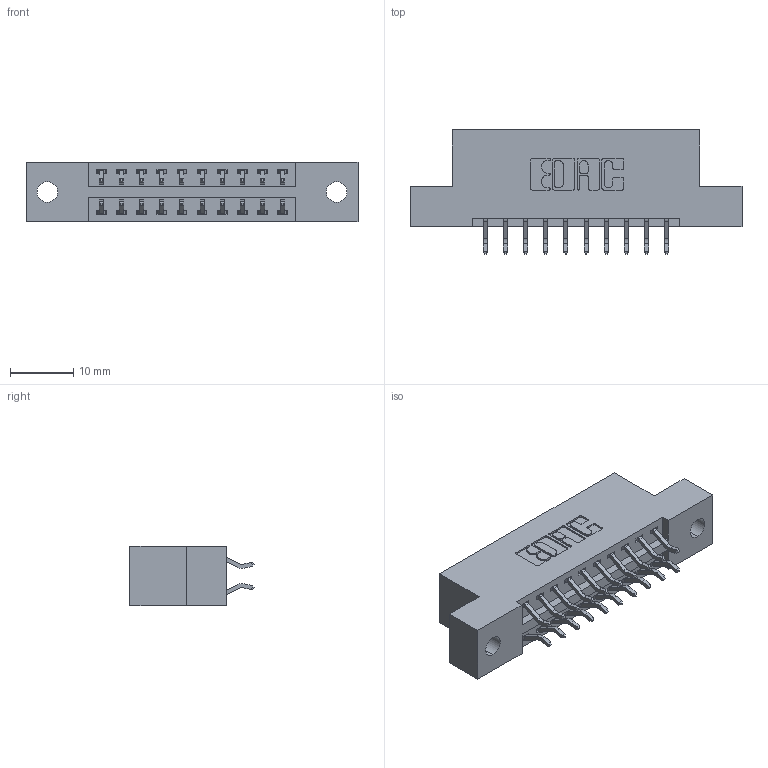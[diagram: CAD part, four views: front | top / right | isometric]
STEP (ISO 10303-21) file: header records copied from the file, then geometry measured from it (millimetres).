
FILE_DESCRIPTION (( 'STEP AP203' ), '1' );
FILE_NAME ('346-020-556-202.STEP', '2022-05-18T19:44:54', ( '' ), ( '' ), 'SwSTEP 2.0', 'SolidWorks 2020', '' );
FILE_SCHEMA (( 'CONFIG_CONTROL_DESIGN' ));
Length unit declared in the file: inch
Products named in the file (3): 346-020-556-202; 346 Part_Flush Mounting Lugs - 0.128 Dia; 345-292-001_556 Tail
Assembly tree (21 placements, depth 2):
  346-020-556-202
    346 Part_Flush Mounting Lugs - 0.128 Dia
    345-292-001_556 Tail  x20
Bounding box: 52.32 x 19.57 x 9.4 mm (x, y, z)
Volume: 179.2 mm3; surface area: 5826.8 mm2
Topology: 20 solids, 21 shells, 1281 faces, 3789 edges, 2498 vertices
Faces by surface type: plane 856, cylinder 425
Entity records: 11057 total; most frequent: CARTESIAN_POINT 1880, ORIENTED_EDGE 1802, DIRECTION 1697, EDGE_CURVE 901, LINE 721, VECTOR 721, VERTEX_POINT 598, AXIS2_PLACEMENT_3D 488
